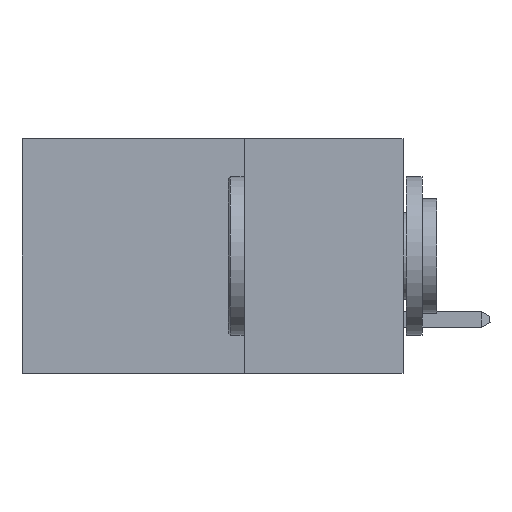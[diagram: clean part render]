
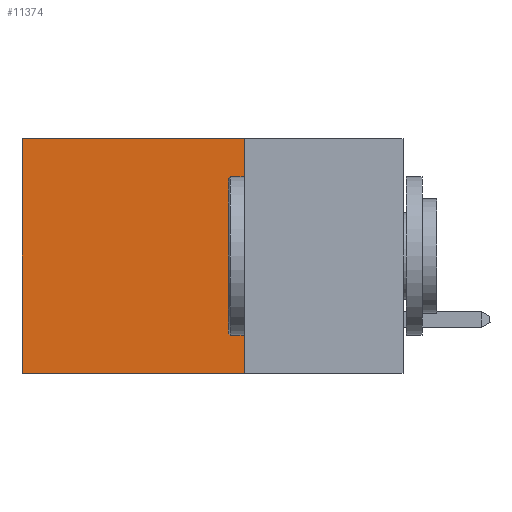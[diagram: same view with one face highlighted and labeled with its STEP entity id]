
A CAD part, left-side view. The second image highlights one B-rep face of the part: STEP entity #11374.
In plain terms, the highlighted planar face has unit normal (-1, 0, 0).
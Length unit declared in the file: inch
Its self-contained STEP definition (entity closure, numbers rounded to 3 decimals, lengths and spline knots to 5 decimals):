
#171 = VERTEX_POINT ( 'NONE', #1544 ) ;
#496 = DIRECTION ( 'NONE',  ( 0., 1., 0. ) ) ;
#1544 = CARTESIAN_POINT ( 'NONE',  ( 0.2875, 0.25, 0. ) ) ;
#3757 = CARTESIAN_POINT ( 'NONE',  ( 0.2875, 0.25, -0.37 ) ) ;
#5124 = LINE ( 'NONE', #40355, #12782 ) ;
#5272 = CARTESIAN_POINT ( 'NONE',  ( 0.2875, 0.6, 0. ) ) ;
#6419 = VECTOR ( 'NONE', #32714, 39.37008 ) ;
#7930 = VERTEX_POINT ( 'NONE', #33335 ) ;
#8176 = ORIENTED_EDGE ( 'NONE', *, *, #28964, .T. ) ;
#10857 = DIRECTION ( 'NONE',  ( 0., 0., -1. ) ) ;
#11374 = ADVANCED_FACE ( 'NONE', ( #28668 ), #16967, .F. ) ;
#12031 = LINE ( 'NONE', #3757, #21725 ) ;
#12034 = VERTEX_POINT ( 'NONE', #5272 ) ;
#12753 = EDGE_LOOP ( 'NONE', ( #15148, #24068, #40702, #8176 ) ) ;
#12782 = VECTOR ( 'NONE', #40225, 39.37008 ) ;
#15148 = ORIENTED_EDGE ( 'NONE', *, *, #33823, .T. ) ;
#15918 = CARTESIAN_POINT ( 'NONE',  ( 0.2875, 0.25, 0. ) ) ;
#16761 = VERTEX_POINT ( 'NONE', #30420 ) ;
#16967 = PLANE ( 'NONE',  #20556 ) ;
#18860 = EDGE_CURVE ( 'NONE', #171, #16761, #27318, .T. ) ;
#18948 = LINE ( 'NONE', #41520, #23058 ) ;
#18961 = EDGE_CURVE ( 'NONE', #16761, #7930, #12031, .T. ) ;
#20397 = DIRECTION ( 'NONE',  ( 1., 0., 0. ) ) ;
#20556 = AXIS2_PLACEMENT_3D ( 'NONE', #23728, #20397, #10857 ) ;
#21725 = VECTOR ( 'NONE', #496, 39.37008 ) ;
#23058 = VECTOR ( 'NONE', #28481, 39.37008 ) ;
#23728 = CARTESIAN_POINT ( 'NONE',  ( 0.2875, 0.25, 0. ) ) ;
#24068 = ORIENTED_EDGE ( 'NONE', *, *, #18961, .F. ) ;
#27318 = LINE ( 'NONE', #15918, #6419 ) ;
#28481 = DIRECTION ( 'NONE',  ( 0., 0., -1. ) ) ;
#28668 = FACE_OUTER_BOUND ( 'NONE', #12753, .T. ) ;
#28964 = EDGE_CURVE ( 'NONE', #171, #12034, #5124, .T. ) ;
#30420 = CARTESIAN_POINT ( 'NONE',  ( 0.2875, 0.25, -0.37 ) ) ;
#32714 = DIRECTION ( 'NONE',  ( 0., 0., -1. ) ) ;
#33335 = CARTESIAN_POINT ( 'NONE',  ( 0.2875, 0.6, -0.37 ) ) ;
#33823 = EDGE_CURVE ( 'NONE', #12034, #7930, #18948, .T. ) ;
#40225 = DIRECTION ( 'NONE',  ( 0., 1., 0. ) ) ;
#40355 = CARTESIAN_POINT ( 'NONE',  ( 0.2875, 0.25, 0. ) ) ;
#40702 = ORIENTED_EDGE ( 'NONE', *, *, #18860, .F. ) ;
#41520 = CARTESIAN_POINT ( 'NONE',  ( 0.2875, 0.6, 0. ) ) ;
